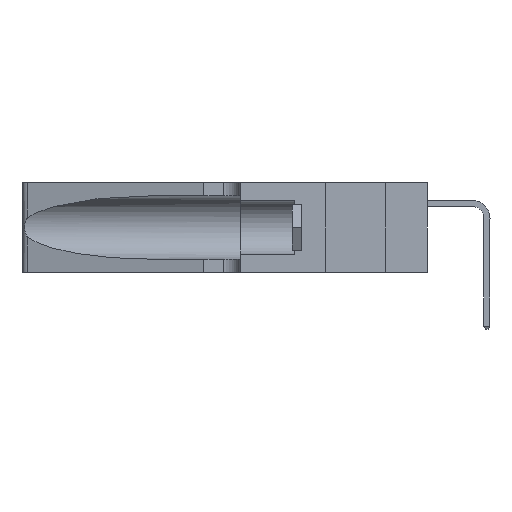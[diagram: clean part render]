
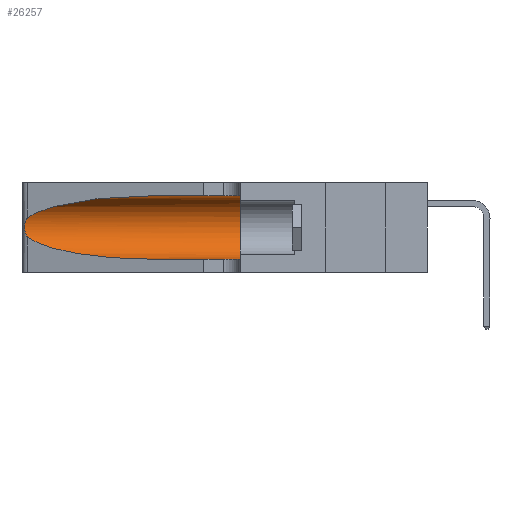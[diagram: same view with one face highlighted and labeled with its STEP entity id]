
A CAD part, left-side view. The second image highlights one B-rep face of the part: STEP entity #26257.
In plain terms, the highlighted cylindrical face has radius 3.308 mm (diameter 6.617 mm), a partial arc.
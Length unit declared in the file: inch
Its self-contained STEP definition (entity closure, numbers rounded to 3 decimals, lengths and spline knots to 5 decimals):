
#93 = EDGE_CURVE ( 'NONE', #28819, #30441, #27276, .T. ) ;
#314 = VERTEX_POINT ( 'NONE', #34759 ) ;
#1208 = EDGE_LOOP ( 'NONE', ( #17832, #35567, #21588, #22976, #25785, #34783 ) ) ;
#2491 = CARTESIAN_POINT ( 'NONE',  ( 0.26075, 1.23896, 0.19203 ) ) ;
#3105 = CIRCLE ( 'NONE', #15965, 0.13025 ) ;
#4180 = VERTEX_POINT ( 'NONE', #24109 ) ;
#4327 = CARTESIAN_POINT ( 'NONE',  ( 0.25487, 1.22718, 0.22369 ) ) ;
#4955 = EDGE_CURVE ( 'NONE', #314, #4180, #37972, .T. ) ;
#5228 = DIRECTION ( 'NONE',  ( 0., -1., 0. ) ) ;
#5642 = CARTESIAN_POINT ( 'NONE',  ( 0.26017, 1.23833, 0.17102 ) ) ;
#5945 = FACE_OUTER_BOUND ( 'NONE', #1208, .T. ) ;
#6218 = CARTESIAN_POINT ( 'NONE',  ( 0.1305, 0.35, 0.185 ) ) ;
#8288 = CARTESIAN_POINT ( 'NONE',  ( 0.1305, 1.61858, 0.185 ) ) ;
#8705 = CARTESIAN_POINT ( 'NONE',  ( 0.25789, 1.23486, 0.15765 ) ) ;
#9291 = DIRECTION ( 'NONE',  ( 0., 0., 1. ) ) ;
#9878 = VERTEX_POINT ( 'NONE', #35852 ) ;
#10487 = LINE ( 'NONE', #25730, #19347 ) ;
#10490 = EDGE_CURVE ( 'NONE', #4180, #32375, #10487, .T. ) ;
#10621 = VECTOR ( 'NONE', #16176, 39.37008 ) ;
#11734 = CARTESIAN_POINT ( 'NONE',  ( 0.25555, 1.22993, 0.14849 ) ) ;
#12459 = EDGE_CURVE ( 'NONE', #9878, #314, #13541, .T. ) ;
#13541 = B_SPLINE_CURVE_WITH_KNOTS ( 'NONE', 3,
 ( #23412, #26363, #35013, #17599, #37910, #20606, #2491, #23543, #5642, #26483, #8705, #29371, #11734, #32258 ),
 .UNSPECIFIED., .F., .F.,
 ( 4, 2, 2, 2, 2, 2, 4 ),
 ( 0., 0.00027, 0.00053, 0.00107, 0.0016, 0.00187, 0.00214 ),
 .UNSPECIFIED. ) ;
#14751 = AXIS2_PLACEMENT_3D ( 'NONE', #8288, #5228, #26099 ) ;
#15641 = CARTESIAN_POINT ( 'NONE',  ( 0.1305, 0.35, 0.05475 ) ) ;
#15652 = CARTESIAN_POINT ( 'NONE',  ( 0.1305, 0.72297, 0.31525 ) ) ;
#15965 = AXIS2_PLACEMENT_3D ( 'NONE', #6218, #27035, #9291 ) ;
#16176 = DIRECTION ( 'NONE',  ( 0., -1., 0. ) ) ;
#16991 = EDGE_CURVE ( 'NONE', #30441, #32375, #3105, .T. ) ;
#17294 = CARTESIAN_POINT ( 'NONE',  ( 0.1305, 0.72297, 0.05475 ) ) ;
#17599 = CARTESIAN_POINT ( 'NONE',  ( 0.25787, 1.23484, 0.2124 ) ) ;
#17832 = ORIENTED_EDGE ( 'NONE', *, *, #19068, .T. ) ;
#19068 = EDGE_CURVE ( 'NONE', #28819, #9878, #25001, .T. ) ;
#19186 = CARTESIAN_POINT ( 'NONE',  ( 0.1305, 1.61858, 0.31525 ) ) ;
#19327 = CARTESIAN_POINT ( 'NONE',  ( 0.18966, 0.96281, 0.31525 ) ) ;
#19347 = VECTOR ( 'NONE', #34264, 39.37008 ) ;
#20606 = CARTESIAN_POINT ( 'NONE',  ( 0.26018, 1.23835, 0.19895 ) ) ;
#21588 = ORIENTED_EDGE ( 'NONE', *, *, #4955, .T. ) ;
#22293 = CARTESIAN_POINT ( 'NONE',  ( 0.2373, 1.15595, 0.28018 ) ) ;
#22976 = ORIENTED_EDGE ( 'NONE', *, *, #10490, .T. ) ;
#23412 = CARTESIAN_POINT ( 'NONE',  ( 0.25487, 1.22718, 0.22369 ) ) ;
#23543 = CARTESIAN_POINT ( 'NONE',  ( 0.26075, 1.23896, 0.178 ) ) ;
#23604 = CARTESIAN_POINT ( 'NONE',  ( 0.1305, 0.35, 0.31525 ) ) ;
#24109 = CARTESIAN_POINT ( 'NONE',  ( 0.1305, 0.72297, 0.05475 ) ) ;
#25001 =( BOUNDED_CURVE ( )  B_SPLINE_CURVE ( 3, ( #36690, #19327, #22293, #4327 ),
 .UNSPECIFIED., .F., .F. ) 
 B_SPLINE_CURVE_WITH_KNOTS ( ( 4, 4 ),
 ( 1.5708, 2.84003 ),
 .UNSPECIFIED. ) 
 CURVE ( )  GEOMETRIC_REPRESENTATION_ITEM ( )  RATIONAL_B_SPLINE_CURVE ( ( 1., 0.87, 0.87, 1. ) ) 
 REPRESENTATION_ITEM ( '' )  );
#25730 = CARTESIAN_POINT ( 'NONE',  ( 0.1305, 1.61858, 0.05475 ) ) ;
#25785 = ORIENTED_EDGE ( 'NONE', *, *, #16991, .F. ) ;
#26099 = DIRECTION ( 'NONE',  ( 0., 0., -1. ) ) ;
#26257 = ADVANCED_FACE ( 'NONE', ( #5945 ), #27793, .F. ) ;
#26363 = CARTESIAN_POINT ( 'NONE',  ( 0.25555, 1.22994, 0.2215 ) ) ;
#26483 = CARTESIAN_POINT ( 'NONE',  ( 0.25856, 1.23593, 0.16098 ) ) ;
#27035 = DIRECTION ( 'NONE',  ( 0., 1., 0. ) ) ;
#27276 = LINE ( 'NONE', #19186, #10621 ) ;
#27793 = CYLINDRICAL_SURFACE ( 'NONE', #14751, 0.13025 ) ;
#28819 = VERTEX_POINT ( 'NONE', #15652 ) ;
#28957 = CARTESIAN_POINT ( 'NONE',  ( 0.2373, 1.15595, 0.08982 ) ) ;
#29371 = CARTESIAN_POINT ( 'NONE',  ( 0.25639, 1.23186, 0.15144 ) ) ;
#30441 = VERTEX_POINT ( 'NONE', #23604 ) ;
#31854 = CARTESIAN_POINT ( 'NONE',  ( 0.25487, 1.22718, 0.14631 ) ) ;
#32258 = CARTESIAN_POINT ( 'NONE',  ( 0.25487, 1.22718, 0.14631 ) ) ;
#32375 = VERTEX_POINT ( 'NONE', #15641 ) ;
#34264 = DIRECTION ( 'NONE',  ( 0., -1., 0. ) ) ;
#34720 = CARTESIAN_POINT ( 'NONE',  ( 0.18966, 0.96281, 0.05475 ) ) ;
#34759 = CARTESIAN_POINT ( 'NONE',  ( 0.25487, 1.22718, 0.14631 ) ) ;
#34783 = ORIENTED_EDGE ( 'NONE', *, *, #93, .F. ) ;
#35013 = CARTESIAN_POINT ( 'NONE',  ( 0.25639, 1.23184, 0.21858 ) ) ;
#35567 = ORIENTED_EDGE ( 'NONE', *, *, #12459, .T. ) ;
#35852 = CARTESIAN_POINT ( 'NONE',  ( 0.25487, 1.22718, 0.22369 ) ) ;
#36690 = CARTESIAN_POINT ( 'NONE',  ( 0.1305, 0.72297, 0.31525 ) ) ;
#37910 = CARTESIAN_POINT ( 'NONE',  ( 0.25854, 1.2359, 0.20912 ) ) ;
#37972 =( BOUNDED_CURVE ( )  B_SPLINE_CURVE ( 3, ( #31854, #28957, #34720, #17294 ),
 .UNSPECIFIED., .F., .F. ) 
 B_SPLINE_CURVE_WITH_KNOTS ( ( 4, 4 ),
 ( 3.44316, 4.71239 ),
 .UNSPECIFIED. ) 
 CURVE ( )  GEOMETRIC_REPRESENTATION_ITEM ( )  RATIONAL_B_SPLINE_CURVE ( ( 1., 0.87, 0.87, 1. ) ) 
 REPRESENTATION_ITEM ( '' )  );
